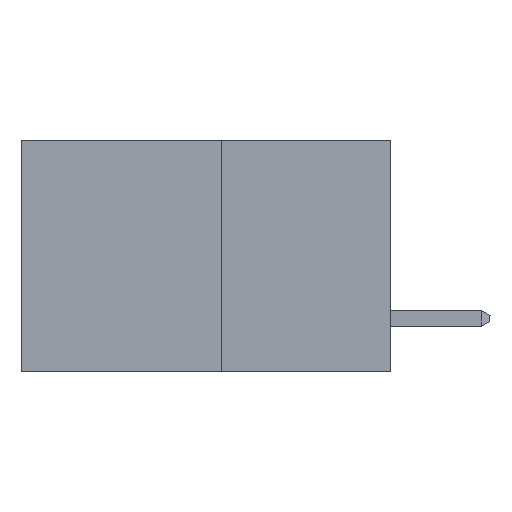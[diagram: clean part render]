
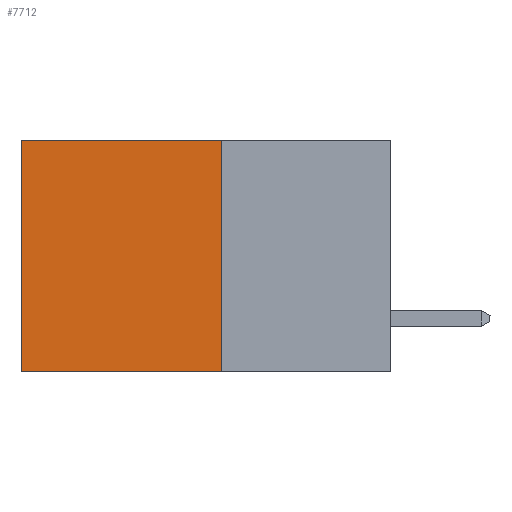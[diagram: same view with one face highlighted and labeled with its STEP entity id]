
A CAD part, left-side view. The second image highlights one B-rep face of the part: STEP entity #7712.
In plain terms, the highlighted planar face has unit normal (-1, 0, 0).
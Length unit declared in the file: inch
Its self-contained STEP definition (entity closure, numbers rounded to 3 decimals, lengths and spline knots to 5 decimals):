
#8 = VERTEX_POINT ( 'NONE', #2387 ) ;
#259 = DIRECTION ( 'NONE',  ( 0., 0., -1. ) ) ;
#461 = VECTOR ( 'NONE', #1972, 39.37008 ) ;
#737 = VERTEX_POINT ( 'NONE', #7419 ) ;
#854 = FACE_OUTER_BOUND ( 'NONE', #4329, .T. ) ;
#895 = VECTOR ( 'NONE', #1824, 39.37008 ) ;
#943 = ORIENTED_EDGE ( 'NONE', *, *, #6303, .T. ) ;
#1824 = DIRECTION ( 'NONE',  ( 0., 0., -1. ) ) ;
#1972 = DIRECTION ( 'NONE',  ( 0., 0., -1. ) ) ;
#2060 = EDGE_CURVE ( 'NONE', #737, #2070, #6890, .T. ) ;
#2070 = VERTEX_POINT ( 'NONE', #9440 ) ;
#2250 = VERTEX_POINT ( 'NONE', #8568 ) ;
#2387 = CARTESIAN_POINT ( 'NONE',  ( 0.277, 0.59, 0. ) ) ;
#3157 = EDGE_CURVE ( 'NONE', #2250, #737, #3737, .T. ) ;
#3737 = LINE ( 'NONE', #6808, #461 ) ;
#4114 = VECTOR ( 'NONE', #9456, 39.37008 ) ;
#4329 = EDGE_LOOP ( 'NONE', ( #5557, #5851, #8043, #943 ) ) ;
#5270 = CARTESIAN_POINT ( 'NONE',  ( 0.277, 0.27, 0. ) ) ;
#5557 = ORIENTED_EDGE ( 'NONE', *, *, #6063, .T. ) ;
#5851 = ORIENTED_EDGE ( 'NONE', *, *, #2060, .F. ) ;
#6063 = EDGE_CURVE ( 'NONE', #8, #2070, #10029, .T. ) ;
#6114 = DIRECTION ( 'NONE',  ( 1., 0., 0. ) ) ;
#6303 = EDGE_CURVE ( 'NONE', #2250, #8, #6947, .T. ) ;
#6808 = CARTESIAN_POINT ( 'NONE',  ( 0.277, 0.27, -0.37 ) ) ;
#6890 = LINE ( 'NONE', #9424, #4114 ) ;
#6947 = LINE ( 'NONE', #5270, #8697 ) ;
#7358 = AXIS2_PLACEMENT_3D ( 'NONE', #10799, #6114, #259 ) ;
#7419 = CARTESIAN_POINT ( 'NONE',  ( 0.277, 0.27, -0.37 ) ) ;
#7443 = CARTESIAN_POINT ( 'NONE',  ( 0.277, 0.59, -0.37 ) ) ;
#7712 = ADVANCED_FACE ( 'NONE', ( #854 ), #10027, .F. ) ;
#8043 = ORIENTED_EDGE ( 'NONE', *, *, #3157, .F. ) ;
#8568 = CARTESIAN_POINT ( 'NONE',  ( 0.277, 0.27, 0. ) ) ;
#8697 = VECTOR ( 'NONE', #10886, 39.37008 ) ;
#9424 = CARTESIAN_POINT ( 'NONE',  ( 0.277, 0.27, -0.37 ) ) ;
#9440 = CARTESIAN_POINT ( 'NONE',  ( 0.277, 0.59, -0.37 ) ) ;
#9456 = DIRECTION ( 'NONE',  ( 0., 1., 0. ) ) ;
#10027 = PLANE ( 'NONE',  #7358 ) ;
#10029 = LINE ( 'NONE', #7443, #895 ) ;
#10799 = CARTESIAN_POINT ( 'NONE',  ( 0.277, 0.27, -0.37 ) ) ;
#10886 = DIRECTION ( 'NONE',  ( 0., 1., 0. ) ) ;
